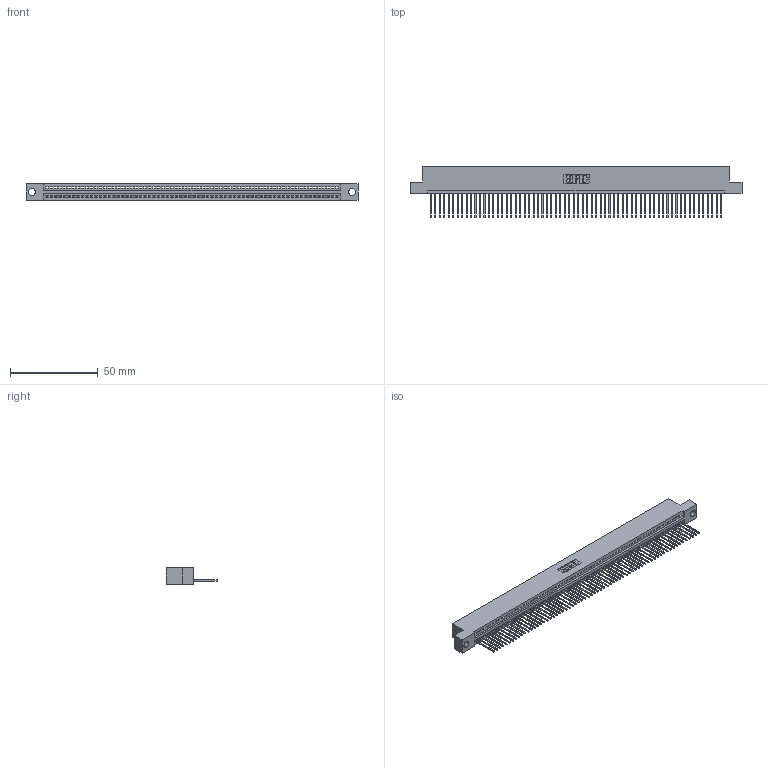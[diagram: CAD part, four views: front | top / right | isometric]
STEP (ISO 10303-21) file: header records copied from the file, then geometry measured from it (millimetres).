
FILE_DESCRIPTION (( 'STEP AP203' ), '1' );
FILE_NAME ('395-066-540-104.STEP', '2021-05-31T22:06:15', ( '' ), ( '' ), 'SwSTEP 2.0', 'SolidWorks 2020', '' );
FILE_SCHEMA (( 'CONFIG_CONTROL_DESIGN' ));
Length unit declared in the file: inch
Products named in the file (3): 345-292-001_345-293-140; 395-066-540-104; 345 Part_Flush Mounting Lugs - 0.156 Dia-TI
Assembly tree (67 placements, depth 2):
  395-066-540-104
    345 Part_Flush Mounting Lugs - 0.156 Dia-TI
    345-292-001_345-293-140  x66
Bounding box: 188.85 x 29.13 x 9.4 mm (x, y, z)
Volume: 18117.1 mm3; surface area: 24887.7 mm2
Topology: 67 solids, 67 shells, 3968 faces, 11993 edges, 7906 vertices
Faces by surface type: plane 2734, cylinder 1234
Entity records: 46879 total; most frequent: CARTESIAN_POINT 8128, ORIENTED_EDGE 8126, DIRECTION 7063, EDGE_CURVE 4063, VECTOR 3667, LINE 3667, VERTEX_POINT 2706, AXIS2_PLACEMENT_3D 1698
